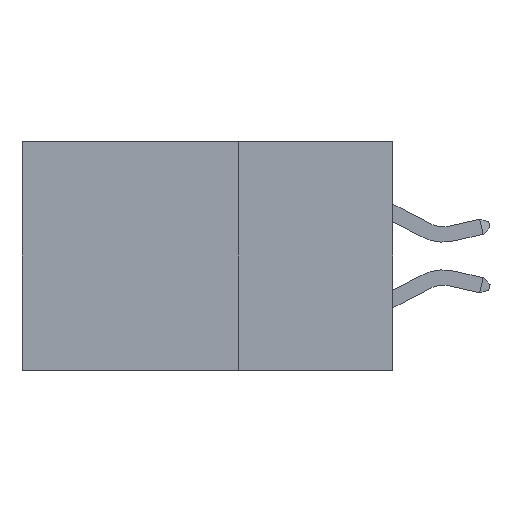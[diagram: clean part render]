
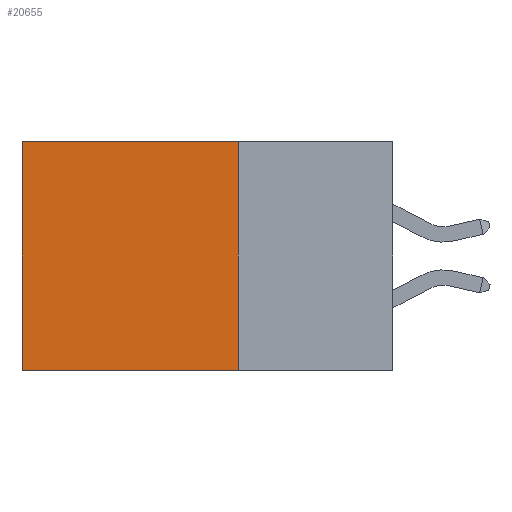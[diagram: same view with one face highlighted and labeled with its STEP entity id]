
A CAD part, left-side view. The second image highlights one B-rep face of the part: STEP entity #20655.
In plain terms, the highlighted planar face has unit normal (-1, 0, 0).
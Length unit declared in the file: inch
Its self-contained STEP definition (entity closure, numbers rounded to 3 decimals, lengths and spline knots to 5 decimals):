
#180 = VECTOR ( 'NONE', #31264, 39.37008 ) ;
#2147 = CARTESIAN_POINT ( 'NONE',  ( 0.2875, 0.6, -0.37 ) ) ;
#2772 = VECTOR ( 'NONE', #16031, 39.37008 ) ;
#3661 = AXIS2_PLACEMENT_3D ( 'NONE', #5885, #16271, #32390 ) ;
#3692 = CARTESIAN_POINT ( 'NONE',  ( 0.2875, 0.25, 0. ) ) ;
#4381 = LINE ( 'NONE', #10099, #180 ) ;
#5885 = CARTESIAN_POINT ( 'NONE',  ( 0.2875, 0.25, 0. ) ) ;
#7243 = ORIENTED_EDGE ( 'NONE', *, *, #23936, .T. ) ;
#7323 = ORIENTED_EDGE ( 'NONE', *, *, #20742, .F. ) ;
#8300 = CARTESIAN_POINT ( 'NONE',  ( 0.2875, 0.25, -0.37 ) ) ;
#8759 = CARTESIAN_POINT ( 'NONE',  ( 0.2875, 0.25, 0. ) ) ;
#9143 = VECTOR ( 'NONE', #20181, 39.37008 ) ;
#9950 = LINE ( 'NONE', #33508, #9143 ) ;
#10099 = CARTESIAN_POINT ( 'NONE',  ( 0.2875, 0.6, 0. ) ) ;
#16003 = LINE ( 'NONE', #8300, #2772 ) ;
#16031 = DIRECTION ( 'NONE',  ( 0., 1., 0. ) ) ;
#16271 = DIRECTION ( 'NONE',  ( 1., 0., 0. ) ) ;
#16363 = LINE ( 'NONE', #8759, #24262 ) ;
#16950 = EDGE_CURVE ( 'NONE', #33196, #24430, #9950, .T. ) ;
#18822 = DIRECTION ( 'NONE',  ( 0., 0., -1. ) ) ;
#18889 = CARTESIAN_POINT ( 'NONE',  ( 0.2875, 0.6, 0. ) ) ;
#19965 = EDGE_CURVE ( 'NONE', #25560, #25942, #16003, .T. ) ;
#20181 = DIRECTION ( 'NONE',  ( 0., 1., 0. ) ) ;
#20655 = ADVANCED_FACE ( 'NONE', ( #21354 ), #21609, .F. ) ;
#20742 = EDGE_CURVE ( 'NONE', #33196, #25560, #16363, .T. ) ;
#21354 = FACE_OUTER_BOUND ( 'NONE', #31166, .T. ) ;
#21609 = PLANE ( 'NONE',  #3661 ) ;
#23936 = EDGE_CURVE ( 'NONE', #24430, #25942, #4381, .T. ) ;
#24262 = VECTOR ( 'NONE', #18822, 39.37008 ) ;
#24328 = ORIENTED_EDGE ( 'NONE', *, *, #16950, .T. ) ;
#24430 = VERTEX_POINT ( 'NONE', #18889 ) ;
#25288 = CARTESIAN_POINT ( 'NONE',  ( 0.2875, 0.25, -0.37 ) ) ;
#25560 = VERTEX_POINT ( 'NONE', #25288 ) ;
#25942 = VERTEX_POINT ( 'NONE', #2147 ) ;
#27185 = ORIENTED_EDGE ( 'NONE', *, *, #19965, .F. ) ;
#31166 = EDGE_LOOP ( 'NONE', ( #7243, #27185, #7323, #24328 ) ) ;
#31264 = DIRECTION ( 'NONE',  ( 0., 0., -1. ) ) ;
#32390 = DIRECTION ( 'NONE',  ( 0., 0., -1. ) ) ;
#33196 = VERTEX_POINT ( 'NONE', #3692 ) ;
#33508 = CARTESIAN_POINT ( 'NONE',  ( 0.2875, 0.25, 0. ) ) ;
